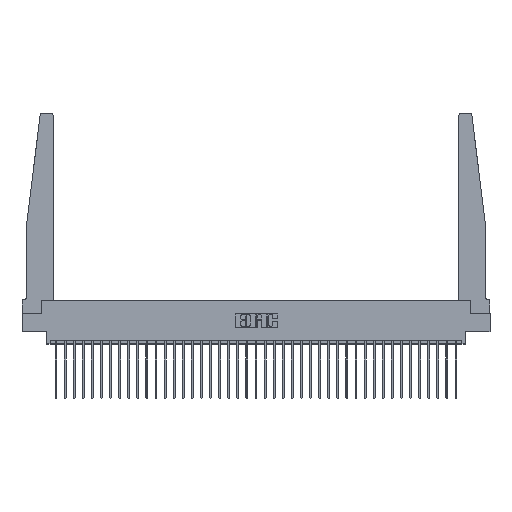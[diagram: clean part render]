
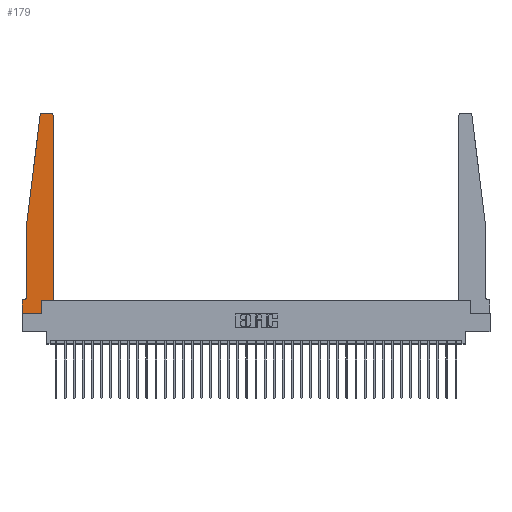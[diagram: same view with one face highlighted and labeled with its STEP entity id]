
A CAD part, top view. The second image highlights one B-rep face of the part: STEP entity #179.
In plain terms, the highlighted planar face has unit normal (0, 0, 1).
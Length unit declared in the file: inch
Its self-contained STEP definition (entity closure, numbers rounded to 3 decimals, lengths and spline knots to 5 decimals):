
#179 = ADVANCED_FACE ( 'NONE', ( #26512 ), #33492, .T. ) ;
#921 = CARTESIAN_POINT ( 'NONE',  ( 0.065, 0.2375, 0.37 ) ) ;
#1109 = VERTEX_POINT ( 'NONE', #25963 ) ;
#1419 = ORIENTED_EDGE ( 'NONE', *, *, #28325, .T. ) ;
#1520 = DIRECTION ( 'NONE',  ( 1., 0., 0. ) ) ;
#1572 = DIRECTION ( 'NONE',  ( -1., 0., 0. ) ) ;
#2241 = DIRECTION ( 'NONE',  ( 1., 0., 0. ) ) ;
#2503 = EDGE_CURVE ( 'NONE', #13462, #21598, #14540, .T. ) ;
#2709 = VERTEX_POINT ( 'NONE', #6522 ) ;
#2781 = AXIS2_PLACEMENT_3D ( 'NONE', #33593, #17918, #2241 ) ;
#2822 = CARTESIAN_POINT ( 'NONE',  ( 0.015, 0.2375, 0.37 ) ) ;
#3696 = LINE ( 'NONE', #26188, #23764 ) ;
#3787 = DIRECTION ( 'NONE',  ( 0., 0., 1. ) ) ;
#5017 = ORIENTED_EDGE ( 'NONE', *, *, #9129, .T. ) ;
#5466 = DIRECTION ( 'NONE',  ( -1., 0., 0. ) ) ;
#5840 = CARTESIAN_POINT ( 'NONE',  ( 0.425, 0.18, 0.37 ) ) ;
#5958 = CARTESIAN_POINT ( 'NONE',  ( 0.2605, 0., 0.37 ) ) ;
#6427 = LINE ( 'NONE', #9487, #11792 ) ;
#6522 = CARTESIAN_POINT ( 'NONE',  ( 0.27653, 2.75, 0.37 ) ) ;
#6665 = VERTEX_POINT ( 'NONE', #9911 ) ;
#6845 = LINE ( 'NONE', #33789, #33860 ) ;
#7499 = ORIENTED_EDGE ( 'NONE', *, *, #16738, .T. ) ;
#8252 = CARTESIAN_POINT ( 'NONE',  ( 0.425, 0.18, 0.37 ) ) ;
#8394 = VECTOR ( 'NONE', #23916, 39.37008 ) ;
#8454 = CARTESIAN_POINT ( 'NONE',  ( 0., 0., 0.37 ) ) ;
#8471 = DIRECTION ( 'NONE',  ( 0., 1., 0. ) ) ;
#8871 = DIRECTION ( 'NONE',  ( 1., 0., 0. ) ) ;
#9129 = EDGE_CURVE ( 'NONE', #12160, #27961, #27792, .T. ) ;
#9487 = CARTESIAN_POINT ( 'NONE',  ( 0.065, 0.1875, 0.37 ) ) ;
#9632 = DIRECTION ( 'NONE',  ( 0., 1., 0. ) ) ;
#9911 = CARTESIAN_POINT ( 'NONE',  ( 0.065, 1.25, 0.37 ) ) ;
#9998 = CARTESIAN_POINT ( 'NONE',  ( 0.015, 0.1875, 0.37 ) ) ;
#10992 = EDGE_LOOP ( 'NONE', ( #7499, #24889, #26207, #11287, #5017, #1419, #11503, #28433, #21689, #17326, #20004, #22664 ) ) ;
#11287 = ORIENTED_EDGE ( 'NONE', *, *, #17593, .T. ) ;
#11494 = CARTESIAN_POINT ( 'NONE',  ( 0., 0.1875, 0.37 ) ) ;
#11503 = ORIENTED_EDGE ( 'NONE', *, *, #29964, .T. ) ;
#11731 = CIRCLE ( 'NONE', #18079, 0.03 ) ;
#11792 = VECTOR ( 'NONE', #1572, 39.37008 ) ;
#12160 = VERTEX_POINT ( 'NONE', #921 ) ;
#12366 = DIRECTION ( 'NONE',  ( -1., 0., 0. ) ) ;
#12837 = EDGE_CURVE ( 'NONE', #21598, #26160, #28082, .T. ) ;
#13341 = VECTOR ( 'NONE', #8471, 39.37008 ) ;
#13462 = VERTEX_POINT ( 'NONE', #21456 ) ;
#14257 = LINE ( 'NONE', #28022, #27363 ) ;
#14345 = CARTESIAN_POINT ( 'NONE',  ( 0.425, 2.72, 0.37 ) ) ;
#14463 = LINE ( 'NONE', #30565, #19774 ) ;
#14540 = LINE ( 'NONE', #8252, #8394 ) ;
#15226 = EDGE_CURVE ( 'NONE', #20157, #19261, #3696, .T. ) ;
#15364 = DIRECTION ( 'NONE',  ( -0.122, -0.992, 0. ) ) ;
#15726 = CARTESIAN_POINT ( 'NONE',  ( 0., 0., 0.37 ) ) ;
#15910 = CARTESIAN_POINT ( 'NONE',  ( 0.065, 1.25, 0.37 ) ) ;
#16738 = EDGE_CURVE ( 'NONE', #28474, #2709, #14257, .T. ) ;
#17183 = DIRECTION ( 'NONE',  ( 0., 0., 1. ) ) ;
#17326 = ORIENTED_EDGE ( 'NONE', *, *, #2503, .T. ) ;
#17454 = EDGE_CURVE ( 'NONE', #28597, #6665, #6845, .T. ) ;
#17593 = EDGE_CURVE ( 'NONE', #6665, #12160, #17950, .T. ) ;
#17918 = DIRECTION ( 'NONE',  ( 0., 0., 1. ) ) ;
#17950 = LINE ( 'NONE', #15910, #31067 ) ;
#18079 = AXIS2_PLACEMENT_3D ( 'NONE', #32878, #17183, #1520 ) ;
#18286 = CARTESIAN_POINT ( 'NONE',  ( 0.24675, 2.72367, 0.37 ) ) ;
#18408 = DIRECTION ( 'NONE',  ( 1., 0., 0. ) ) ;
#18562 = DIRECTION ( 'NONE',  ( 0., -1., 0. ) ) ;
#18805 = EDGE_CURVE ( 'NONE', #26160, #28474, #11731, .T. ) ;
#19261 = VERTEX_POINT ( 'NONE', #5958 ) ;
#19774 = VECTOR ( 'NONE', #9632, 39.37008 ) ;
#19821 = VECTOR ( 'NONE', #29410, 39.37008 ) ;
#20004 = ORIENTED_EDGE ( 'NONE', *, *, #12837, .T. ) ;
#20157 = VERTEX_POINT ( 'NONE', #15726 ) ;
#21124 = DIRECTION ( 'NONE',  ( 0., 0., -1. ) ) ;
#21162 = EDGE_CURVE ( 'NONE', #19261, #13462, #14463, .T. ) ;
#21240 = CARTESIAN_POINT ( 'NONE',  ( 0.425, 0.18, 0.37 ) ) ;
#21456 = CARTESIAN_POINT ( 'NONE',  ( 0.2605, 0.18, 0.37 ) ) ;
#21598 = VERTEX_POINT ( 'NONE', #21240 ) ;
#21689 = ORIENTED_EDGE ( 'NONE', *, *, #21162, .T. ) ;
#22664 = ORIENTED_EDGE ( 'NONE', *, *, #18805, .T. ) ;
#23764 = VECTOR ( 'NONE', #18408, 39.37008 ) ;
#23916 = DIRECTION ( 'NONE',  ( 1., 0., 0. ) ) ;
#24889 = ORIENTED_EDGE ( 'NONE', *, *, #33652, .T. ) ;
#25963 = CARTESIAN_POINT ( 'NONE',  ( 0., 0.1875, 0.37 ) ) ;
#26160 = VERTEX_POINT ( 'NONE', #14345 ) ;
#26188 = CARTESIAN_POINT ( 'NONE',  ( 0., 0., 0.37 ) ) ;
#26207 = ORIENTED_EDGE ( 'NONE', *, *, #17454, .T. ) ;
#26512 = FACE_OUTER_BOUND ( 'NONE', #10992, .T. ) ;
#27363 = VECTOR ( 'NONE', #12366, 39.37008 ) ;
#27792 = CIRCLE ( 'NONE', #30832, 0.05 ) ;
#27961 = VERTEX_POINT ( 'NONE', #9998 ) ;
#28022 = CARTESIAN_POINT ( 'NONE',  ( 0.25, 2.75, 0.37 ) ) ;
#28082 = LINE ( 'NONE', #5840, #13341 ) ;
#28325 = EDGE_CURVE ( 'NONE', #27961, #1109, #6427, .T. ) ;
#28393 = CARTESIAN_POINT ( 'NONE',  ( 0.395, 2.75, 0.37 ) ) ;
#28433 = ORIENTED_EDGE ( 'NONE', *, *, #15226, .T. ) ;
#28474 = VERTEX_POINT ( 'NONE', #28393 ) ;
#28597 = VERTEX_POINT ( 'NONE', #18286 ) ;
#29410 = DIRECTION ( 'NONE',  ( 0., -1., 0. ) ) ;
#29964 = EDGE_CURVE ( 'NONE', #1109, #20157, #33754, .T. ) ;
#30565 = CARTESIAN_POINT ( 'NONE',  ( 0.2605, 0.18, 0.37 ) ) ;
#30832 = AXIS2_PLACEMENT_3D ( 'NONE', #2822, #21124, #5466 ) ;
#31067 = VECTOR ( 'NONE', #18562, 39.37008 ) ;
#31405 = CIRCLE ( 'NONE', #2781, 0.03 ) ;
#32878 = CARTESIAN_POINT ( 'NONE',  ( 0.395, 2.72, 0.37 ) ) ;
#33492 = PLANE ( 'NONE',  #33703 ) ;
#33593 = CARTESIAN_POINT ( 'NONE',  ( 0.27653, 2.72, 0.37 ) ) ;
#33652 = EDGE_CURVE ( 'NONE', #2709, #28597, #31405, .T. ) ;
#33703 = AXIS2_PLACEMENT_3D ( 'NONE', #11494, #3787, #8871 ) ;
#33754 = LINE ( 'NONE', #8454, #19821 ) ;
#33789 = CARTESIAN_POINT ( 'NONE',  ( 0.065, 1.25, 0.37 ) ) ;
#33860 = VECTOR ( 'NONE', #15364, 39.37008 ) ;
